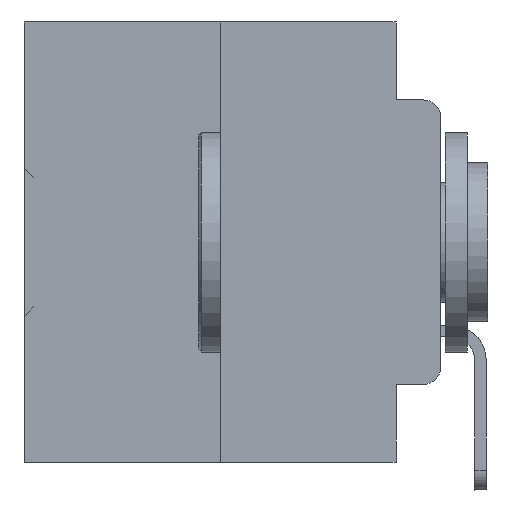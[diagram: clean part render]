
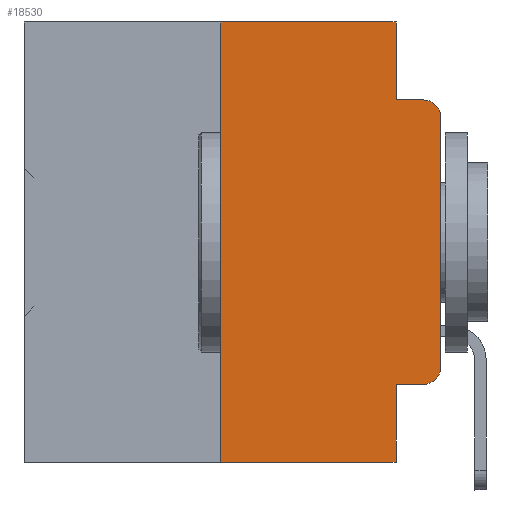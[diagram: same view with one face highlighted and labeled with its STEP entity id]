
A CAD part, left-side view. The second image highlights one B-rep face of the part: STEP entity #18530.
In plain terms, the highlighted planar face has unit normal (-1, 0, 0).
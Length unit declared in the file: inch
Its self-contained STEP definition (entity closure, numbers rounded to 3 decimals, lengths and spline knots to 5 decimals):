
#620 = VERTEX_POINT ( 'NONE', #30715 ) ;
#1140 = AXIS2_PLACEMENT_3D ( 'NONE', #38345, #26424, #11549 ) ;
#2085 = ORIENTED_EDGE ( 'NONE', *, *, #20663, .F. ) ;
#2222 = DIRECTION ( 'NONE',  ( 0., -1., 0. ) ) ;
#2877 = CARTESIAN_POINT ( 'NONE',  ( 0., 0., 0. ) ) ;
#3233 = FACE_OUTER_BOUND ( 'NONE', #32617, .T. ) ;
#4313 = EDGE_CURVE ( 'NONE', #36345, #27947, #37650, .T. ) ;
#4712 = CARTESIAN_POINT ( 'NONE',  ( 0., 0.051, -0.0885 ) ) ;
#4783 = VECTOR ( 'NONE', #8167, 39.37008 ) ;
#7487 = EDGE_CURVE ( 'NONE', #22182, #11815, #10204, .T. ) ;
#8167 = DIRECTION ( 'NONE',  ( 0., 0., 1. ) ) ;
#8342 = EDGE_CURVE ( 'NONE', #22182, #34777, #34514, .T. ) ;
#8373 = DIRECTION ( 'NONE',  ( 0., 0., -1. ) ) ;
#9088 = EDGE_CURVE ( 'NONE', #28017, #32890, #23434, .T. ) ;
#9207 = EDGE_CURVE ( 'NONE', #620, #12019, #15198, .T. ) ;
#9318 = CARTESIAN_POINT ( 'NONE',  ( 0., 0.473, 0. ) ) ;
#9575 = CARTESIAN_POINT ( 'NONE',  ( 0., 0., -0.1085 ) ) ;
#9893 = DIRECTION ( 'NONE',  ( 0., 0., -1. ) ) ;
#9918 = CARTESIAN_POINT ( 'NONE',  ( 0., 0.051, 0. ) ) ;
#10037 = VECTOR ( 'NONE', #8373, 39.37008 ) ;
#10075 = VECTOR ( 'NONE', #15272, 39.37008 ) ;
#10204 = LINE ( 'NONE', #19206, #24799 ) ;
#10291 = EDGE_CURVE ( 'NONE', #27947, #28017, #14866, .T. ) ;
#11172 = LINE ( 'NONE', #4712, #15988 ) ;
#11549 = DIRECTION ( 'NONE',  ( 0., 0., -1. ) ) ;
#11787 = ORIENTED_EDGE ( 'NONE', *, *, #9088, .T. ) ;
#11815 = VERTEX_POINT ( 'NONE', #17802 ) ;
#11900 = LINE ( 'NONE', #23442, #10037 ) ;
#12006 = CARTESIAN_POINT ( 'NONE',  ( 0., 0.051, -0.4115 ) ) ;
#12019 = VERTEX_POINT ( 'NONE', #23266 ) ;
#12686 = CARTESIAN_POINT ( 'NONE',  ( 0., 0.02, -0.0885 ) ) ;
#13778 = CARTESIAN_POINT ( 'NONE',  ( 0., 0.473, -0.5 ) ) ;
#14866 = CIRCLE ( 'NONE', #1140, 0.02 ) ;
#15198 = LINE ( 'NONE', #9918, #35421 ) ;
#15272 = DIRECTION ( 'NONE',  ( 0., -1., 0. ) ) ;
#15784 = DIRECTION ( 'NONE',  ( 0., 0., -1. ) ) ;
#15988 = VECTOR ( 'NONE', #25473, 39.37008 ) ;
#16035 = CARTESIAN_POINT ( 'NONE',  ( 0., 0., -0.3915 ) ) ;
#16204 = AXIS2_PLACEMENT_3D ( 'NONE', #9318, #21834, #9893 ) ;
#17303 = CARTESIAN_POINT ( 'NONE',  ( 0., 0.051, -0.4115 ) ) ;
#17435 = DIRECTION ( 'NONE',  ( -1., 0., 0. ) ) ;
#17802 = CARTESIAN_POINT ( 'NONE',  ( 0., 0.25, 0. ) ) ;
#17952 = ORIENTED_EDGE ( 'NONE', *, *, #4313, .T. ) ;
#18530 = ADVANCED_FACE ( 'NONE', ( #3233 ), #36681, .F. ) ;
#19099 = ORIENTED_EDGE ( 'NONE', *, *, #27777, .F. ) ;
#19206 = CARTESIAN_POINT ( 'NONE',  ( 0., 0.25, 0. ) ) ;
#19773 = VERTEX_POINT ( 'NONE', #12686 ) ;
#19994 = DIRECTION ( 'NONE',  ( 0., 0., -1. ) ) ;
#20184 = CARTESIAN_POINT ( 'NONE',  ( 0., 0.02, -0.1085 ) ) ;
#20234 = ORIENTED_EDGE ( 'NONE', *, *, #7487, .F. ) ;
#20663 = EDGE_CURVE ( 'NONE', #11815, #620, #29964, .T. ) ;
#21834 = DIRECTION ( 'NONE',  ( 1., 0., 0. ) ) ;
#22146 = DIRECTION ( 'NONE',  ( 0., 0., 1. ) ) ;
#22182 = VERTEX_POINT ( 'NONE', #36972 ) ;
#23266 = CARTESIAN_POINT ( 'NONE',  ( 0., 0.051, -0.0885 ) ) ;
#23434 = LINE ( 'NONE', #2877, #4783 ) ;
#23442 = CARTESIAN_POINT ( 'NONE',  ( 0., 0.051, 0. ) ) ;
#23491 = CARTESIAN_POINT ( 'NONE',  ( 0., 0.02, -0.4115 ) ) ;
#24799 = VECTOR ( 'NONE', #22146, 39.37008 ) ;
#25473 = DIRECTION ( 'NONE',  ( 0., -1., 0. ) ) ;
#26424 = DIRECTION ( 'NONE',  ( -1., 0., 0. ) ) ;
#27046 = ORIENTED_EDGE ( 'NONE', *, *, #10291, .T. ) ;
#27777 = EDGE_CURVE ( 'NONE', #12019, #19773, #11172, .T. ) ;
#27947 = VERTEX_POINT ( 'NONE', #23491 ) ;
#28017 = VERTEX_POINT ( 'NONE', #16035 ) ;
#28346 = VECTOR ( 'NONE', #28858, 39.37008 ) ;
#28858 = DIRECTION ( 'NONE',  ( 0., -1., 0. ) ) ;
#28995 = EDGE_CURVE ( 'NONE', #32890, #19773, #33515, .T. ) ;
#29224 = ORIENTED_EDGE ( 'NONE', *, *, #8342, .T. ) ;
#29964 = LINE ( 'NONE', #33267, #10075 ) ;
#30715 = CARTESIAN_POINT ( 'NONE',  ( 0., 0.051, 0. ) ) ;
#32617 = EDGE_LOOP ( 'NONE', ( #11787, #37711, #19099, #37329, #2085, #20234, #29224, #33076, #17952, #27046 ) ) ;
#32890 = VERTEX_POINT ( 'NONE', #9575 ) ;
#33076 = ORIENTED_EDGE ( 'NONE', *, *, #34134, .F. ) ;
#33267 = CARTESIAN_POINT ( 'NONE',  ( 0., 0.473, 0. ) ) ;
#33515 = CIRCLE ( 'NONE', #36025, 0.02 ) ;
#34134 = EDGE_CURVE ( 'NONE', #36345, #34777, #11900, .T. ) ;
#34240 = VECTOR ( 'NONE', #2222, 39.37008 ) ;
#34514 = LINE ( 'NONE', #13778, #34240 ) ;
#34777 = VERTEX_POINT ( 'NONE', #36480 ) ;
#35421 = VECTOR ( 'NONE', #15784, 39.37008 ) ;
#36025 = AXIS2_PLACEMENT_3D ( 'NONE', #20184, #17435, #19994 ) ;
#36345 = VERTEX_POINT ( 'NONE', #12006 ) ;
#36480 = CARTESIAN_POINT ( 'NONE',  ( 0., 0.051, -0.5 ) ) ;
#36681 = PLANE ( 'NONE',  #16204 ) ;
#36972 = CARTESIAN_POINT ( 'NONE',  ( 0., 0.25, -0.5 ) ) ;
#37329 = ORIENTED_EDGE ( 'NONE', *, *, #9207, .F. ) ;
#37650 = LINE ( 'NONE', #17303, #28346 ) ;
#37711 = ORIENTED_EDGE ( 'NONE', *, *, #28995, .T. ) ;
#38345 = CARTESIAN_POINT ( 'NONE',  ( 0., 0.02, -0.3915 ) ) ;
